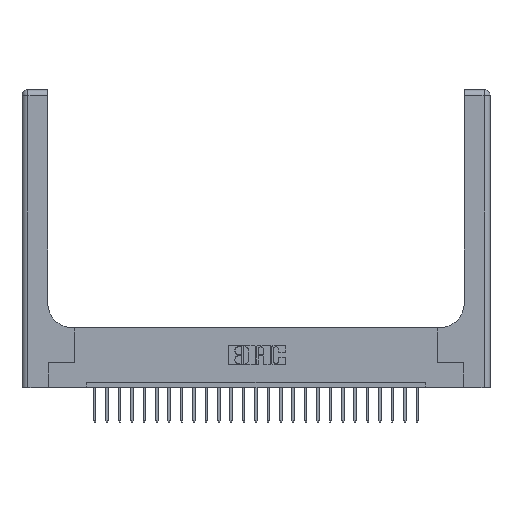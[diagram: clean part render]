
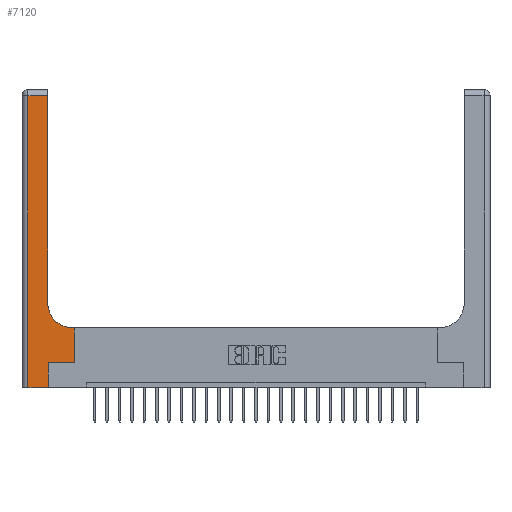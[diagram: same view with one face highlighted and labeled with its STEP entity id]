
A CAD part, top view. The second image highlights one B-rep face of the part: STEP entity #7120.
In plain terms, the highlighted planar face has unit normal (0, 0, 1).
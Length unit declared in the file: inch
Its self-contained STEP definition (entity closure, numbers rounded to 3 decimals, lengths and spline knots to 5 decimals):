
#92 = VECTOR ( 'NONE', #1403, 39.37008 ) ;
#287 = CARTESIAN_POINT ( 'NONE',  ( 0.265, 0.25, 0.37 ) ) ;
#744 = ORIENTED_EDGE ( 'NONE', *, *, #837, .T. ) ;
#837 = EDGE_CURVE ( 'NONE', #10612, #6138, #10719, .T. ) ;
#1064 = CARTESIAN_POINT ( 'NONE',  ( 0.26, 3., 0.37 ) ) ;
#1361 = DIRECTION ( 'NONE',  ( 0., 1., 0. ) ) ;
#1403 = DIRECTION ( 'NONE',  ( 0., 1., 0. ) ) ;
#1476 = CARTESIAN_POINT ( 'NONE',  ( 0.26, 0.85, 0.37 ) ) ;
#1568 = DIRECTION ( 'NONE',  ( 0., 0., -1. ) ) ;
#1875 = EDGE_CURVE ( 'NONE', #2723, #2356, #20231, .T. ) ;
#2356 = VERTEX_POINT ( 'NONE', #22681 ) ;
#2676 = ORIENTED_EDGE ( 'NONE', *, *, #8118, .T. ) ;
#2723 = VERTEX_POINT ( 'NONE', #15526 ) ;
#3104 = VERTEX_POINT ( 'NONE', #16348 ) ;
#3257 = ORIENTED_EDGE ( 'NONE', *, *, #21586, .T. ) ;
#3752 = CARTESIAN_POINT ( 'NONE',  ( 0.26, 0.6, 0.37 ) ) ;
#3942 = EDGE_CURVE ( 'NONE', #3104, #10612, #18631, .T. ) ;
#4636 = ORIENTED_EDGE ( 'NONE', *, *, #6208, .T. ) ;
#4737 = DIRECTION ( 'NONE',  ( 0., 0., -1. ) ) ;
#4814 = VECTOR ( 'NONE', #1361, 39.37008 ) ;
#5107 = CARTESIAN_POINT ( 'NONE',  ( 0., 2.94, 0.37 ) ) ;
#5196 = VECTOR ( 'NONE', #8649, 39.37008 ) ;
#6138 = VERTEX_POINT ( 'NONE', #18319 ) ;
#6173 = CARTESIAN_POINT ( 'NONE',  ( 0., 0., 0.37 ) ) ;
#6208 = EDGE_CURVE ( 'NONE', #2356, #12069, #13611, .T. ) ;
#6367 = CARTESIAN_POINT ( 'NONE',  ( 0.528, 0.6, 0.37 ) ) ;
#6538 = PLANE ( 'NONE',  #19382 ) ;
#6571 = LINE ( 'NONE', #21683, #4814 ) ;
#6711 = VECTOR ( 'NONE', #11405, 39.37008 ) ;
#6978 = DIRECTION ( 'NONE',  ( -1., 0., 0. ) ) ;
#7120 = ADVANCED_FACE ( 'NONE', ( #19925 ), #6538, .F. ) ;
#8118 = EDGE_CURVE ( 'NONE', #17821, #2723, #12930, .T. ) ;
#8649 = DIRECTION ( 'NONE',  ( 0., 1., 0. ) ) ;
#9001 = CARTESIAN_POINT ( 'NONE',  ( 0.51, 0.85, 0.37 ) ) ;
#9260 = EDGE_CURVE ( 'NONE', #15468, #17821, #16445, .T. ) ;
#10015 = EDGE_CURVE ( 'NONE', #6138, #15468, #10072, .T. ) ;
#10072 = CIRCLE ( 'NONE', #11772, 0.25 ) ;
#10301 = ORIENTED_EDGE ( 'NONE', *, *, #10015, .T. ) ;
#10612 = VERTEX_POINT ( 'NONE', #6367 ) ;
#10719 = LINE ( 'NONE', #3752, #13035 ) ;
#10890 = CARTESIAN_POINT ( 'NONE',  ( 0.26, 2.94, 0.37 ) ) ;
#11090 = EDGE_CURVE ( 'NONE', #12069, #12033, #6571, .T. ) ;
#11405 = DIRECTION ( 'NONE',  ( 1., 0., 0. ) ) ;
#11772 = AXIS2_PLACEMENT_3D ( 'NONE', #9001, #1568, #23893 ) ;
#12033 = VERTEX_POINT ( 'NONE', #287 ) ;
#12069 = VERTEX_POINT ( 'NONE', #18911 ) ;
#12092 = CARTESIAN_POINT ( 'NONE',  ( 0., 3., 0.37 ) ) ;
#12496 = VECTOR ( 'NONE', #15331, 39.37008 ) ;
#12510 = CARTESIAN_POINT ( 'NONE',  ( 0.528, 0.25, 0.37 ) ) ;
#12588 = ORIENTED_EDGE ( 'NONE', *, *, #9260, .T. ) ;
#12930 = LINE ( 'NONE', #5107, #17563 ) ;
#13035 = VECTOR ( 'NONE', #14987, 39.37008 ) ;
#13611 = LINE ( 'NONE', #6173, #6711 ) ;
#14838 = ORIENTED_EDGE ( 'NONE', *, *, #11090, .T. ) ;
#14918 = CARTESIAN_POINT ( 'NONE',  ( 0.06, 3., 0.37 ) ) ;
#14987 = DIRECTION ( 'NONE',  ( -1., 0., 0. ) ) ;
#15331 = DIRECTION ( 'NONE',  ( 1., 0., 0. ) ) ;
#15468 = VERTEX_POINT ( 'NONE', #1476 ) ;
#15526 = CARTESIAN_POINT ( 'NONE',  ( 0.06, 2.94, 0.37 ) ) ;
#15862 = VECTOR ( 'NONE', #18209, 39.37008 ) ;
#16348 = CARTESIAN_POINT ( 'NONE',  ( 0.528, 0.25, 0.37 ) ) ;
#16445 = LINE ( 'NONE', #1064, #5196 ) ;
#17563 = VECTOR ( 'NONE', #6978, 39.37008 ) ;
#17821 = VERTEX_POINT ( 'NONE', #10890 ) ;
#17988 = ORIENTED_EDGE ( 'NONE', *, *, #3942, .T. ) ;
#18209 = DIRECTION ( 'NONE',  ( 0., -1., 0. ) ) ;
#18319 = CARTESIAN_POINT ( 'NONE',  ( 0.51, 0.6, 0.37 ) ) ;
#18631 = LINE ( 'NONE', #12510, #92 ) ;
#18911 = CARTESIAN_POINT ( 'NONE',  ( 0.265, 0., 0.37 ) ) ;
#19382 = AXIS2_PLACEMENT_3D ( 'NONE', #12092, #4737, #23373 ) ;
#19873 = ORIENTED_EDGE ( 'NONE', *, *, #1875, .T. ) ;
#19925 = FACE_OUTER_BOUND ( 'NONE', #21035, .T. ) ;
#20231 = LINE ( 'NONE', #14918, #15862 ) ;
#20256 = CARTESIAN_POINT ( 'NONE',  ( 0.265, 0.25, 0.37 ) ) ;
#21035 = EDGE_LOOP ( 'NONE', ( #12588, #2676, #19873, #4636, #14838, #3257, #17988, #744, #10301 ) ) ;
#21586 = EDGE_CURVE ( 'NONE', #12033, #3104, #22039, .T. ) ;
#21683 = CARTESIAN_POINT ( 'NONE',  ( 0.265, 0., 0.37 ) ) ;
#22039 = LINE ( 'NONE', #20256, #12496 ) ;
#22681 = CARTESIAN_POINT ( 'NONE',  ( 0.06, 0., 0.37 ) ) ;
#23373 = DIRECTION ( 'NONE',  ( -1., 0., 0. ) ) ;
#23893 = DIRECTION ( 'NONE',  ( 1., 0., 0. ) ) ;
